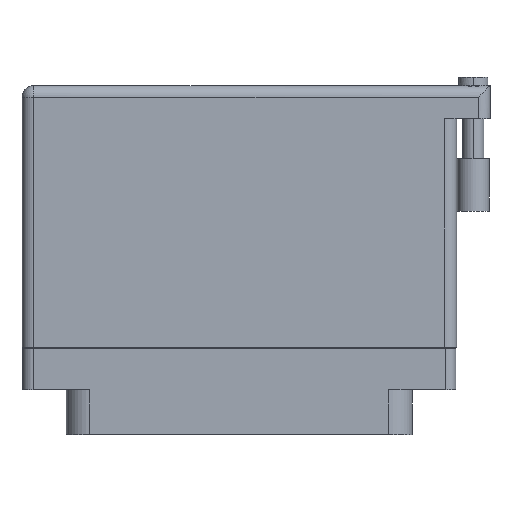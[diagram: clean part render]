
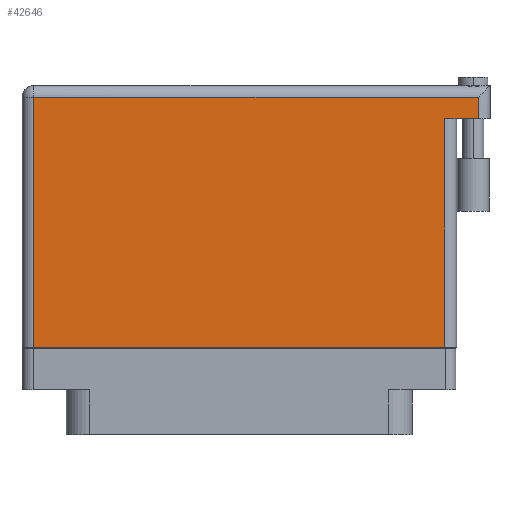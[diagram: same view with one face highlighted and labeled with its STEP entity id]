
A CAD part, front view. The second image highlights one B-rep face of the part: STEP entity #42646.
In plain terms, the highlighted face is planar.
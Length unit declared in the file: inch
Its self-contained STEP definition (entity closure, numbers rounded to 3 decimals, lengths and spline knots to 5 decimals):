
#116 = DIRECTION ( 'NONE',  ( -1., 0., 0. ) ) ;
#291 = DIRECTION ( 'NONE',  ( -1., 0., 0. ) ) ;
#514 = CARTESIAN_POINT ( 'NONE',  ( 1.23, -0.1, 0.4495 ) ) ;
#1672 = DIRECTION ( 'NONE',  ( 0., 1., 0. ) ) ;
#1799 = CARTESIAN_POINT ( 'NONE',  ( -1.23, 1.396, 0.4495 ) ) ;
#1912 = VECTOR ( 'NONE', #35894, 39.37008 ) ;
#3703 = VECTOR ( 'NONE', #116, 39.37008 ) ;
#6859 = ORIENTED_EDGE ( 'NONE', *, *, #8511, .T. ) ;
#7273 = CARTESIAN_POINT ( 'NONE',  ( 1.5, 1.269, 0.4495 ) ) ;
#7644 = LINE ( 'NONE', #11045, #3703 ) ;
#7891 = EDGE_CURVE ( 'NONE', #46739, #47032, #15556, .T. ) ;
#8511 = EDGE_CURVE ( 'NONE', #28612, #39095, #26852, .T. ) ;
#8692 = DIRECTION ( 'NONE',  ( -1., 0., 0. ) ) ;
#10284 = CARTESIAN_POINT ( 'NONE',  ( 1.43, 1.269, 0.4495 ) ) ;
#11045 = CARTESIAN_POINT ( 'NONE',  ( -1.3, 1.396, 0.4495 ) ) ;
#12071 = CARTESIAN_POINT ( 'NONE',  ( -1.3, -0.1, 0.4495 ) ) ;
#14111 = VECTOR ( 'NONE', #45206, 39.37008 ) ;
#15556 = LINE ( 'NONE', #26873, #39577 ) ;
#17511 = EDGE_CURVE ( 'NONE', #47209, #28612, #7644, .T. ) ;
#19321 = PLANE ( 'NONE',  #42701 ) ;
#19743 = EDGE_LOOP ( 'NONE', ( #28334, #43204, #33613, #28705, #42520, #6859 ) ) ;
#21753 = CARTESIAN_POINT ( 'NONE',  ( -1.23, -0.1, 0.4495 ) ) ;
#22339 = DIRECTION ( 'NONE',  ( 0., -1., 0. ) ) ;
#22428 = EDGE_CURVE ( 'NONE', #41066, #47032, #42137, .T. ) ;
#23604 = CARTESIAN_POINT ( 'NONE',  ( -1.3, 1.466, 0.4495 ) ) ;
#24101 = CARTESIAN_POINT ( 'NONE',  ( 1.23, 1.269, 0.4495 ) ) ;
#24827 = CARTESIAN_POINT ( 'NONE',  ( 1.43, 1.466, 0.4495 ) ) ;
#25536 = VECTOR ( 'NONE', #291, 39.37008 ) ;
#26770 = DIRECTION ( 'NONE',  ( 0., 0., -1. ) ) ;
#26852 = LINE ( 'NONE', #41017, #45154 ) ;
#26873 = CARTESIAN_POINT ( 'NONE',  ( 1.23, 1.269, 0.4495 ) ) ;
#28334 = ORIENTED_EDGE ( 'NONE', *, *, #46844, .T. ) ;
#28612 = VERTEX_POINT ( 'NONE', #1799 ) ;
#28705 = ORIENTED_EDGE ( 'NONE', *, *, #42893, .T. ) ;
#28886 = LINE ( 'NONE', #12071, #14111 ) ;
#33613 = ORIENTED_EDGE ( 'NONE', *, *, #22428, .F. ) ;
#35641 = CARTESIAN_POINT ( 'NONE',  ( 1.43, 1.396, 0.4495 ) ) ;
#35894 = DIRECTION ( 'NONE',  ( 0., 1., 0. ) ) ;
#37789 = FACE_OUTER_BOUND ( 'NONE', #19743, .T. ) ;
#39095 = VERTEX_POINT ( 'NONE', #21753 ) ;
#39577 = VECTOR ( 'NONE', #1672, 39.37008 ) ;
#41017 = CARTESIAN_POINT ( 'NONE',  ( -1.23, -0.1, 0.4495 ) ) ;
#41066 = VERTEX_POINT ( 'NONE', #10284 ) ;
#42137 = LINE ( 'NONE', #7273, #25536 ) ;
#42520 = ORIENTED_EDGE ( 'NONE', *, *, #17511, .T. ) ;
#42646 = ADVANCED_FACE ( 'NONE', ( #37789 ), #19321, .F. ) ;
#42701 = AXIS2_PLACEMENT_3D ( 'NONE', #23604, #26770, #8692 ) ;
#42860 = LINE ( 'NONE', #24827, #1912 ) ;
#42893 = EDGE_CURVE ( 'NONE', #41066, #47209, #42860, .T. ) ;
#43204 = ORIENTED_EDGE ( 'NONE', *, *, #7891, .T. ) ;
#45154 = VECTOR ( 'NONE', #22339, 39.37008 ) ;
#45206 = DIRECTION ( 'NONE',  ( 1., 0., 0. ) ) ;
#46739 = VERTEX_POINT ( 'NONE', #514 ) ;
#46844 = EDGE_CURVE ( 'NONE', #39095, #46739, #28886, .T. ) ;
#47032 = VERTEX_POINT ( 'NONE', #24101 ) ;
#47209 = VERTEX_POINT ( 'NONE', #35641 ) ;
